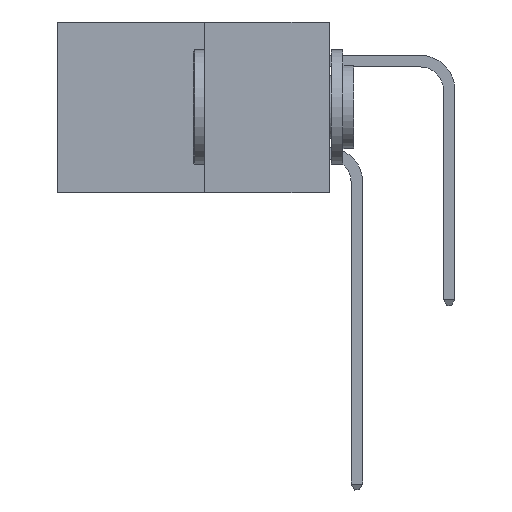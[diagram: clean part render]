
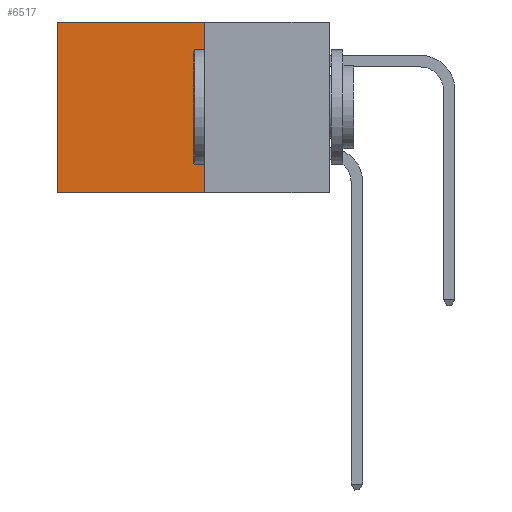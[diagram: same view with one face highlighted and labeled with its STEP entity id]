
A CAD part, left-side view. The second image highlights one B-rep face of the part: STEP entity #6517.
In plain terms, the highlighted planar face has unit normal (-1, 0, 0).
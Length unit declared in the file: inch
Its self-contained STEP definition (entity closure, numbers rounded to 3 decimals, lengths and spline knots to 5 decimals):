
#653 = CARTESIAN_POINT ( 'NONE',  ( 0.277, 0.27, 0. ) ) ;
#910 = DIRECTION ( 'NONE',  ( 0., 0., -1. ) ) ;
#1921 = EDGE_LOOP ( 'NONE', ( #22693, #12747, #14620, #22393 ) ) ;
#3755 = VECTOR ( 'NONE', #910, 39.37008 ) ;
#5555 = LINE ( 'NONE', #12405, #21106 ) ;
#6075 = AXIS2_PLACEMENT_3D ( 'NONE', #7148, #7045, #6989 ) ;
#6517 = ADVANCED_FACE ( 'NONE', ( #20425 ), #7361, .F. ) ;
#6525 = CARTESIAN_POINT ( 'NONE',  ( 0.277, 0.27, -0.37 ) ) ;
#6989 = DIRECTION ( 'NONE',  ( 0., 0., -1. ) ) ;
#7045 = DIRECTION ( 'NONE',  ( 1., 0., 0. ) ) ;
#7148 = CARTESIAN_POINT ( 'NONE',  ( 0.277, 0.27, -0.37 ) ) ;
#7361 = PLANE ( 'NONE',  #6075 ) ;
#7750 = EDGE_CURVE ( 'NONE', #24117, #12079, #14761, .T. ) ;
#8604 = DIRECTION ( 'NONE',  ( 0., 1., 0. ) ) ;
#9037 = DIRECTION ( 'NONE',  ( 0., 1., 0. ) ) ;
#9043 = LINE ( 'NONE', #653, #24410 ) ;
#11301 = CARTESIAN_POINT ( 'NONE',  ( 0.277, 0.27, -0.37 ) ) ;
#12079 = VERTEX_POINT ( 'NONE', #22331 ) ;
#12232 = VERTEX_POINT ( 'NONE', #16879 ) ;
#12405 = CARTESIAN_POINT ( 'NONE',  ( 0.277, 0.59, -0.37 ) ) ;
#12747 = ORIENTED_EDGE ( 'NONE', *, *, #16876, .F. ) ;
#14320 = EDGE_CURVE ( 'NONE', #24117, #23158, #9043, .T. ) ;
#14620 = ORIENTED_EDGE ( 'NONE', *, *, #7750, .F. ) ;
#14761 = LINE ( 'NONE', #11301, #3755 ) ;
#16876 = EDGE_CURVE ( 'NONE', #12079, #12232, #22987, .T. ) ;
#16879 = CARTESIAN_POINT ( 'NONE',  ( 0.277, 0.59, -0.37 ) ) ;
#17412 = EDGE_CURVE ( 'NONE', #23158, #12232, #5555, .T. ) ;
#17758 = VECTOR ( 'NONE', #8604, 39.37008 ) ;
#18775 = CARTESIAN_POINT ( 'NONE',  ( 0.277, 0.27, 0. ) ) ;
#20106 = CARTESIAN_POINT ( 'NONE',  ( 0.277, 0.59, 0. ) ) ;
#20401 = DIRECTION ( 'NONE',  ( 0., 0., -1. ) ) ;
#20425 = FACE_OUTER_BOUND ( 'NONE', #1921, .T. ) ;
#21106 = VECTOR ( 'NONE', #20401, 39.37008 ) ;
#22331 = CARTESIAN_POINT ( 'NONE',  ( 0.277, 0.27, -0.37 ) ) ;
#22393 = ORIENTED_EDGE ( 'NONE', *, *, #14320, .T. ) ;
#22693 = ORIENTED_EDGE ( 'NONE', *, *, #17412, .T. ) ;
#22987 = LINE ( 'NONE', #6525, #17758 ) ;
#23158 = VERTEX_POINT ( 'NONE', #20106 ) ;
#24117 = VERTEX_POINT ( 'NONE', #18775 ) ;
#24410 = VECTOR ( 'NONE', #9037, 39.37008 ) ;
